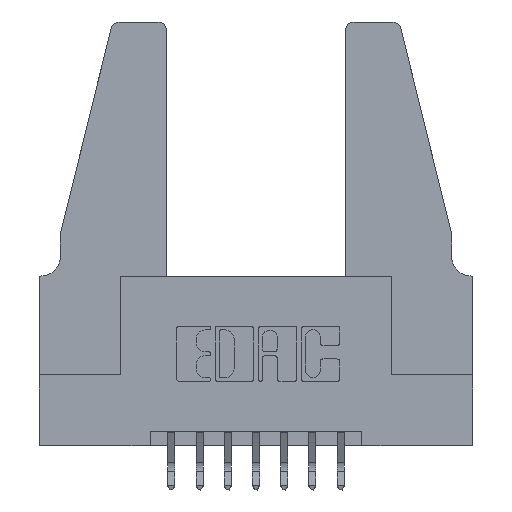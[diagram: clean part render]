
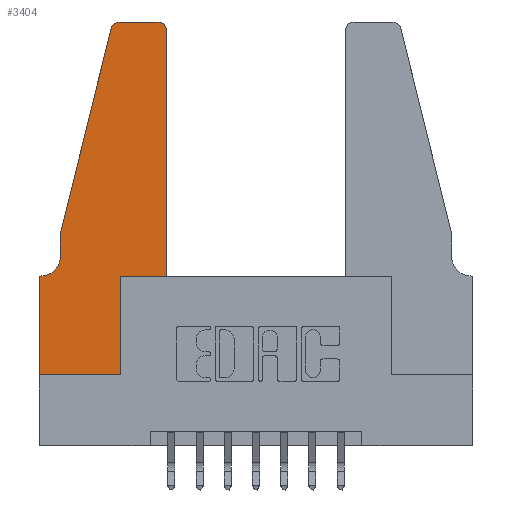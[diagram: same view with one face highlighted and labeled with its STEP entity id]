
A CAD part, top view. The second image highlights one B-rep face of the part: STEP entity #3404.
In plain terms, the highlighted planar face has unit normal (0, 0, 1).
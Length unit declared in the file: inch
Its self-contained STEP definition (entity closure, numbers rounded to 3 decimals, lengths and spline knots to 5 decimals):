
#9 = DIRECTION ( 'NONE',  ( 1., 0., 0. ) ) ;
#12 = DIRECTION ( 'NONE',  ( 0., 0., 1. ) ) ;
#200 = EDGE_CURVE ( 'NONE', #5321, #5614, #6865, .T. ) ;
#354 = DIRECTION ( 'NONE',  ( 1., 0., 0. ) ) ;
#423 = CIRCLE ( 'NONE', #1291, 0.03 ) ;
#502 = DIRECTION ( 'NONE',  ( 0., 0., 1. ) ) ;
#566 = CARTESIAN_POINT ( 'NONE',  ( 0.284, 1.25, 0.37 ) ) ;
#580 = EDGE_CURVE ( 'NONE', #776, #6904, #10769, .T. ) ;
#664 = VERTEX_POINT ( 'NONE', #8745 ) ;
#771 = CIRCLE ( 'NONE', #2133, 0.03 ) ;
#776 = VERTEX_POINT ( 'NONE', #6277 ) ;
#898 = DIRECTION ( 'NONE',  ( -1., 0., 0. ) ) ;
#1084 = CARTESIAN_POINT ( 'NONE',  ( 0.0055, 0.42, 0.37 ) ) ;
#1088 = VERTEX_POINT ( 'NONE', #566 ) ;
#1206 = EDGE_CURVE ( 'NONE', #1088, #664, #423, .T. ) ;
#1291 = AXIS2_PLACEMENT_3D ( 'NONE', #2078, #12, #3107 ) ;
#1311 = ORIENTED_EDGE ( 'NONE', *, *, #4482, .T. ) ;
#1516 = DIRECTION ( 'NONE',  ( -0.239, -0.971, 0. ) ) ;
#2078 = CARTESIAN_POINT ( 'NONE',  ( 0.284, 1.22, 0.37 ) ) ;
#2094 = ORIENTED_EDGE ( 'NONE', *, *, #2339, .T. ) ;
#2110 = LINE ( 'NONE', #10188, #11971 ) ;
#2133 = AXIS2_PLACEMENT_3D ( 'NONE', #9081, #3433, #10041 ) ;
#2153 = DIRECTION ( 'NONE',  ( -1., 0., 0. ) ) ;
#2331 = CARTESIAN_POINT ( 'NONE',  ( 0.4505, 0.35, 0.37 ) ) ;
#2339 = EDGE_CURVE ( 'NONE', #6904, #3377, #11518, .T. ) ;
#2503 = DIRECTION ( 'NONE',  ( 0., 1., 0. ) ) ;
#2619 = DIRECTION ( 'NONE',  ( 0., 1., 0. ) ) ;
#2666 = CARTESIAN_POINT ( 'NONE',  ( 0.0055, 0.35, 0.37 ) ) ;
#2737 = LINE ( 'NONE', #11528, #10057 ) ;
#3000 = AXIS2_PLACEMENT_3D ( 'NONE', #9317, #502, #7475 ) ;
#3016 = EDGE_CURVE ( 'NONE', #3683, #1088, #2737, .T. ) ;
#3041 = CARTESIAN_POINT ( 'NONE',  ( 0., 0., 0.37 ) ) ;
#3044 = ORIENTED_EDGE ( 'NONE', *, *, #10291, .T. ) ;
#3107 = DIRECTION ( 'NONE',  ( 1., 0., 0. ) ) ;
#3144 = VERTEX_POINT ( 'NONE', #9866 ) ;
#3377 = VERTEX_POINT ( 'NONE', #8318 ) ;
#3392 = ORIENTED_EDGE ( 'NONE', *, *, #9468, .T. ) ;
#3404 = ADVANCED_FACE ( 'NONE', ( #10908 ), #3664, .T. ) ;
#3433 = DIRECTION ( 'NONE',  ( 0., 0., 1. ) ) ;
#3436 = AXIS2_PLACEMENT_3D ( 'NONE', #1084, #7945, #2153 ) ;
#3524 = ORIENTED_EDGE ( 'NONE', *, *, #10219, .T. ) ;
#3605 = EDGE_LOOP ( 'NONE', ( #10456, #7110, #7926, #9417, #4301, #3392, #1311, #10036, #3044, #4623, #2094, #3524 ) ) ;
#3664 = PLANE ( 'NONE',  #3000 ) ;
#3683 = VERTEX_POINT ( 'NONE', #12524 ) ;
#3737 = EDGE_CURVE ( 'NONE', #5614, #5259, #9593, .T. ) ;
#4043 = DIRECTION ( 'NONE',  ( -1., 0., 0. ) ) ;
#4301 = ORIENTED_EDGE ( 'NONE', *, *, #3737, .T. ) ;
#4331 = VERTEX_POINT ( 'NONE', #6022 ) ;
#4391 = CARTESIAN_POINT ( 'NONE',  ( 0.0755, 0.5, 0.37 ) ) ;
#4482 = EDGE_CURVE ( 'NONE', #3144, #7913, #5051, .T. ) ;
#4620 = VECTOR ( 'NONE', #7174, 39.37008 ) ;
#4623 = ORIENTED_EDGE ( 'NONE', *, *, #580, .T. ) ;
#5051 = LINE ( 'NONE', #8991, #4620 ) ;
#5259 = VERTEX_POINT ( 'NONE', #2666 ) ;
#5273 = VECTOR ( 'NONE', #2503, 39.37008 ) ;
#5321 = VERTEX_POINT ( 'NONE', #10386 ) ;
#5614 = VERTEX_POINT ( 'NONE', #10774 ) ;
#5660 = VECTOR ( 'NONE', #354, 39.37008 ) ;
#5892 = CARTESIAN_POINT ( 'NONE',  ( 0.4505, 0.35, 0.37 ) ) ;
#5958 = LINE ( 'NONE', #8274, #5660 ) ;
#6022 = CARTESIAN_POINT ( 'NONE',  ( 0.2865, 0., 0.37 ) ) ;
#6277 = CARTESIAN_POINT ( 'NONE',  ( 0.2865, 0.35, 0.37 ) ) ;
#6344 = CARTESIAN_POINT ( 'NONE',  ( 0.4505, 0.35, 0.37 ) ) ;
#6865 = LINE ( 'NONE', #4391, #9321 ) ;
#6904 = VERTEX_POINT ( 'NONE', #6344 ) ;
#7110 = ORIENTED_EDGE ( 'NONE', *, *, #1206, .T. ) ;
#7174 = DIRECTION ( 'NONE',  ( 0., -1., 0. ) ) ;
#7461 = LINE ( 'NONE', #8252, #5273 ) ;
#7475 = DIRECTION ( 'NONE',  ( 1., 0., 0. ) ) ;
#7604 = EDGE_CURVE ( 'NONE', #7913, #4331, #5958, .T. ) ;
#7913 = VERTEX_POINT ( 'NONE', #3041 ) ;
#7926 = ORIENTED_EDGE ( 'NONE', *, *, #10969, .T. ) ;
#7945 = DIRECTION ( 'NONE',  ( 0., 0., -1. ) ) ;
#8252 = CARTESIAN_POINT ( 'NONE',  ( 0.2865, 0.35, 0.37 ) ) ;
#8274 = CARTESIAN_POINT ( 'NONE',  ( 0., 0., 0.37 ) ) ;
#8318 = CARTESIAN_POINT ( 'NONE',  ( 0.4505, 1.22, 0.37 ) ) ;
#8717 = CARTESIAN_POINT ( 'NONE',  ( 0.0755, 0.35, 0.37 ) ) ;
#8745 = CARTESIAN_POINT ( 'NONE',  ( 0.25487, 1.22718, 0.37 ) ) ;
#8991 = CARTESIAN_POINT ( 'NONE',  ( 0., 0., 0.37 ) ) ;
#9081 = CARTESIAN_POINT ( 'NONE',  ( 0.4205, 1.22, 0.37 ) ) ;
#9317 = CARTESIAN_POINT ( 'NONE',  ( 0., 0.35, 0.37 ) ) ;
#9321 = VECTOR ( 'NONE', #10208, 39.37008 ) ;
#9417 = ORIENTED_EDGE ( 'NONE', *, *, #200, .T. ) ;
#9468 = EDGE_CURVE ( 'NONE', #5259, #3144, #9983, .T. ) ;
#9593 = CIRCLE ( 'NONE', #3436, 0.07 ) ;
#9679 = VECTOR ( 'NONE', #4043, 39.37008 ) ;
#9866 = CARTESIAN_POINT ( 'NONE',  ( 0., 0.35, 0.37 ) ) ;
#9983 = LINE ( 'NONE', #8717, #9679 ) ;
#10036 = ORIENTED_EDGE ( 'NONE', *, *, #7604, .T. ) ;
#10041 = DIRECTION ( 'NONE',  ( 1., 0., 0. ) ) ;
#10057 = VECTOR ( 'NONE', #898, 39.37008 ) ;
#10188 = CARTESIAN_POINT ( 'NONE',  ( 0.0755, 0.5, 0.37 ) ) ;
#10205 = VECTOR ( 'NONE', #9, 39.37008 ) ;
#10208 = DIRECTION ( 'NONE',  ( 0., -1., 0. ) ) ;
#10219 = EDGE_CURVE ( 'NONE', #3377, #3683, #771, .T. ) ;
#10291 = EDGE_CURVE ( 'NONE', #4331, #776, #7461, .T. ) ;
#10386 = CARTESIAN_POINT ( 'NONE',  ( 0.0755, 0.5, 0.37 ) ) ;
#10456 = ORIENTED_EDGE ( 'NONE', *, *, #3016, .T. ) ;
#10769 = LINE ( 'NONE', #2331, #10205 ) ;
#10774 = CARTESIAN_POINT ( 'NONE',  ( 0.0755, 0.42, 0.37 ) ) ;
#10908 = FACE_OUTER_BOUND ( 'NONE', #3605, .T. ) ;
#10969 = EDGE_CURVE ( 'NONE', #664, #5321, #2110, .T. ) ;
#11216 = VECTOR ( 'NONE', #2619, 39.37008 ) ;
#11518 = LINE ( 'NONE', #5892, #11216 ) ;
#11528 = CARTESIAN_POINT ( 'NONE',  ( 0.2605, 1.25, 0.37 ) ) ;
#11971 = VECTOR ( 'NONE', #1516, 39.37008 ) ;
#12524 = CARTESIAN_POINT ( 'NONE',  ( 0.4205, 1.25, 0.37 ) ) ;
